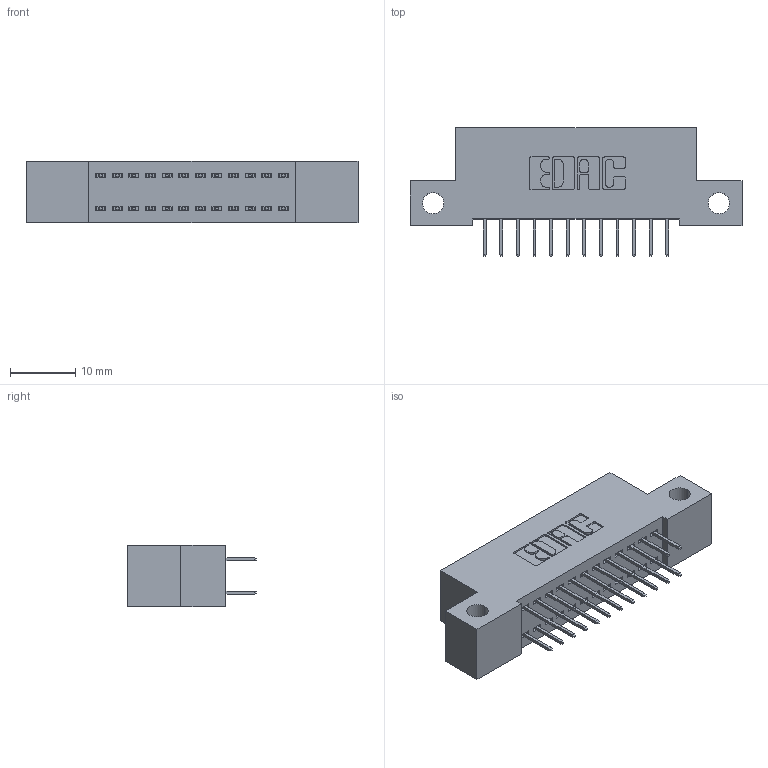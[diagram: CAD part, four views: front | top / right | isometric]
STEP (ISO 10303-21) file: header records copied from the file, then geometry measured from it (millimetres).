
FILE_DESCRIPTION (( 'STEP AP203' ), '1' );
FILE_NAME ('392-024-524-212.STEP', '2018-08-15T13:59:29', ( '' ), ( '' ), 'SwSTEP 2.0', 'SolidWorks 2016', '' );
FILE_SCHEMA (( 'CONFIG_CONTROL_DESIGN' ));
Length unit declared in the file: inch
Products named in the file (3): 342 Part_Side Mount; 345-292-001_345-293-124; 392-024-524-212
Assembly tree (25 placements, depth 2):
  392-024-524-212
    342 Part_Side Mount
    345-292-001_345-293-124  x24
Bounding box: 50.8 x 19.69 x 9.4 mm (x, y, z)
Volume: 4312.1 mm3; surface area: 6025.6 mm2
Topology: 25 solids, 25 shells, 1454 faces, 4115 edges, 2646 vertices
Faces by surface type: plane 1074, cylinder 380
Entity records: 11545 total; most frequent: CARTESIAN_POINT 1946, ORIENTED_EDGE 1882, DIRECTION 1717, EDGE_CURVE 941, VECTOR 817, LINE 817, VERTEX_POINT 622, AXIS2_PLACEMENT_3D 450
